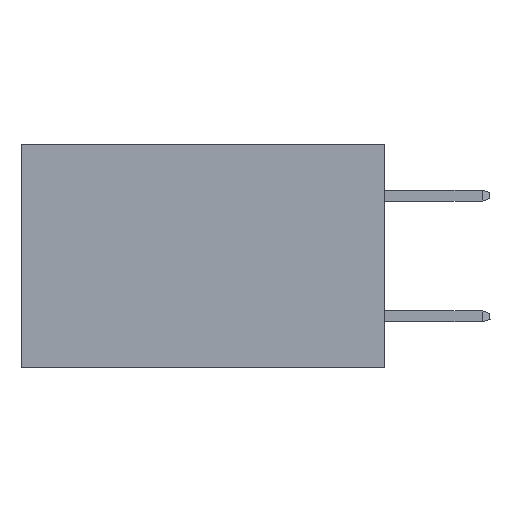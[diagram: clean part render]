
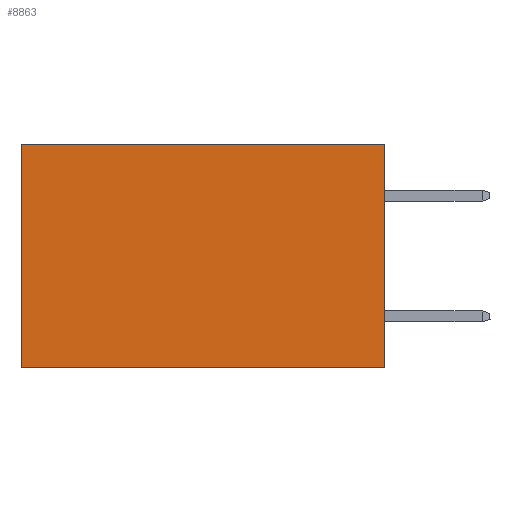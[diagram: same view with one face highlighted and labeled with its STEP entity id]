
A CAD part, left-side view. The second image highlights one B-rep face of the part: STEP entity #8863.
In plain terms, the highlighted planar face has unit normal (-1, 0, 0).
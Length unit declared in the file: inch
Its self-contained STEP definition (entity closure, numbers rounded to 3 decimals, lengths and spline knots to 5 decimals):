
#123 = DIRECTION ( 'NONE',  ( 0., 0., -1. ) ) ;
#186 = CARTESIAN_POINT ( 'NONE',  ( 0.2615, 0.6, -0.37 ) ) ;
#653 = VECTOR ( 'NONE', #8290, 39.37008 ) ;
#708 = VERTEX_POINT ( 'NONE', #3592 ) ;
#1492 = CARTESIAN_POINT ( 'NONE',  ( 0.2615, 0., -0.37 ) ) ;
#1639 = DIRECTION ( 'NONE',  ( 0., 0., -1. ) ) ;
#1698 = VERTEX_POINT ( 'NONE', #2342 ) ;
#1813 = EDGE_CURVE ( 'NONE', #1698, #4257, #5080, .T. ) ;
#2307 = ORIENTED_EDGE ( 'NONE', *, *, #1813, .T. ) ;
#2342 = CARTESIAN_POINT ( 'NONE',  ( 0.2615, 0.6, 0. ) ) ;
#2391 = VERTEX_POINT ( 'NONE', #7307 ) ;
#2930 = EDGE_CURVE ( 'NONE', #708, #1698, #5907, .T. ) ;
#3519 = CARTESIAN_POINT ( 'NONE',  ( 0.2615, 0., -0.37 ) ) ;
#3592 = CARTESIAN_POINT ( 'NONE',  ( 0.2615, 0., 0. ) ) ;
#3836 = ORIENTED_EDGE ( 'NONE', *, *, #2930, .T. ) ;
#4007 = VECTOR ( 'NONE', #1639, 39.37008 ) ;
#4257 = VERTEX_POINT ( 'NONE', #7091 ) ;
#4549 = PLANE ( 'NONE',  #7247 ) ;
#4585 = EDGE_CURVE ( 'NONE', #708, #2391, #6559, .T. ) ;
#4746 = EDGE_LOOP ( 'NONE', ( #2307, #6977, #4802, #3836 ) ) ;
#4802 = ORIENTED_EDGE ( 'NONE', *, *, #4585, .F. ) ;
#5080 = LINE ( 'NONE', #186, #4007 ) ;
#5117 = CARTESIAN_POINT ( 'NONE',  ( 0.2615, 0., -0.37 ) ) ;
#5153 = CARTESIAN_POINT ( 'NONE',  ( 0.2615, 0., 0. ) ) ;
#5268 = DIRECTION ( 'NONE',  ( 1., 0., 0. ) ) ;
#5907 = LINE ( 'NONE', #5153, #7464 ) ;
#6158 = EDGE_CURVE ( 'NONE', #2391, #4257, #8762, .T. ) ;
#6559 = LINE ( 'NONE', #3519, #8879 ) ;
#6977 = ORIENTED_EDGE ( 'NONE', *, *, #6158, .F. ) ;
#7091 = CARTESIAN_POINT ( 'NONE',  ( 0.2615, 0.6, -0.37 ) ) ;
#7247 = AXIS2_PLACEMENT_3D ( 'NONE', #1492, #5268, #123 ) ;
#7307 = CARTESIAN_POINT ( 'NONE',  ( 0.2615, 0., -0.37 ) ) ;
#7323 = DIRECTION ( 'NONE',  ( 0., 0., -1. ) ) ;
#7464 = VECTOR ( 'NONE', #7533, 39.37008 ) ;
#7533 = DIRECTION ( 'NONE',  ( 0., 1., 0. ) ) ;
#8290 = DIRECTION ( 'NONE',  ( 0., 1., 0. ) ) ;
#8762 = LINE ( 'NONE', #5117, #653 ) ;
#8863 = ADVANCED_FACE ( 'NONE', ( #8888 ), #4549, .F. ) ;
#8879 = VECTOR ( 'NONE', #7323, 39.37008 ) ;
#8888 = FACE_OUTER_BOUND ( 'NONE', #4746, .T. ) ;
